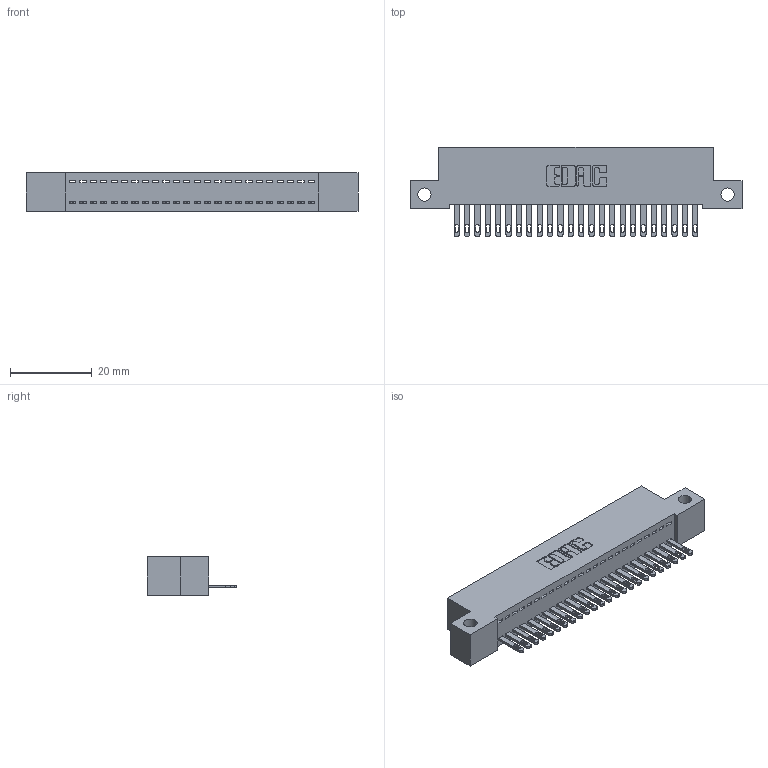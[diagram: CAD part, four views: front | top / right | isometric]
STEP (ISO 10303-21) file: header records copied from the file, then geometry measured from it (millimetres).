
FILE_DESCRIPTION (( 'STEP AP203' ), '1' );
FILE_NAME ('892-024-500-112.STEP', '2020-09-21T14:23:53', ( '' ), ( '' ), 'SwSTEP 2.0', 'SolidWorks 2020', '' );
FILE_SCHEMA (( 'CONFIG_CONTROL_DESIGN' ));
Length unit declared in the file: inch
Products named in the file (3): 892-024-500-112; 842 Part_Side Mount; 345-292-001_345-293-100
Assembly tree (25 placements, depth 2):
  892-024-500-112
    842 Part_Side Mount
    345-292-001_345-293-100  x24
Bounding box: 81.28 x 21.85 x 9.4 mm (x, y, z)
Volume: 7001.3 mm3; surface area: 9829.1 mm2
Topology: 25 solids, 25 shells, 1406 faces, 4331 edges, 2886 vertices
Faces by surface type: plane 930, cylinder 476
Entity records: 16801 total; most frequent: CARTESIAN_POINT 2906, ORIENTED_EDGE 2866, DIRECTION 2489, EDGE_CURVE 1433, LINE 1301, VECTOR 1301, VERTEX_POINT 954, AXIS2_PLACEMENT_3D 594
